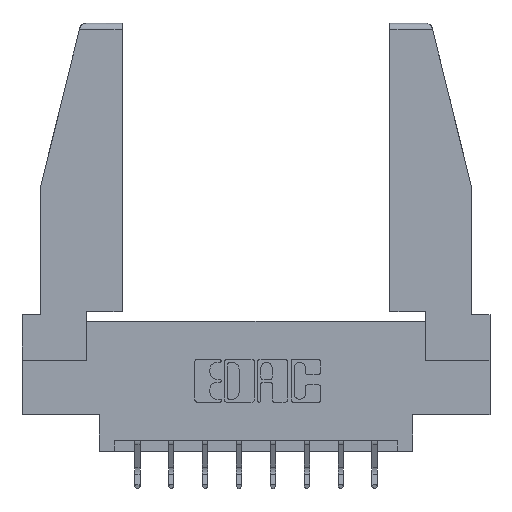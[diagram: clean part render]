
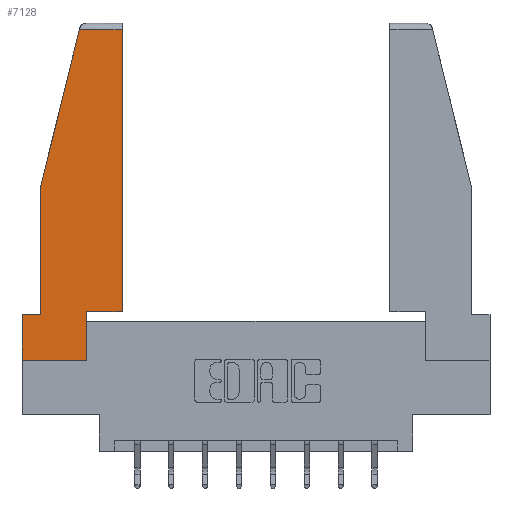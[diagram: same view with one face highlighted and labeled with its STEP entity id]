
A CAD part, top view. The second image highlights one B-rep face of the part: STEP entity #7128.
In plain terms, the highlighted planar face has unit normal (0, 0, 1).
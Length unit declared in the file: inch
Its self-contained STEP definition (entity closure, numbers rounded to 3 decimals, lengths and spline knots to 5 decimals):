
#110 = CARTESIAN_POINT ( 'NONE',  ( 0., 0.21, 0. ) ) ;
#155 = DIRECTION ( 'NONE',  ( 0., 0., 1. ) ) ;
#453 = DIRECTION ( 'NONE',  ( -1., 0., 0. ) ) ;
#784 = LINE ( 'NONE', #9707, #3025 ) ;
#1427 = VECTOR ( 'NONE', #5321, 39.37008 ) ;
#1780 = ORIENTED_EDGE ( 'NONE', *, *, #3735, .T. ) ;
#1814 = CARTESIAN_POINT ( 'NONE',  ( 0.086, 0.8, 0. ) ) ;
#1915 = ORIENTED_EDGE ( 'NONE', *, *, #5568, .T. ) ;
#1966 = CARTESIAN_POINT ( 'NONE',  ( 0.297, 0., 0. ) ) ;
#2128 = CARTESIAN_POINT ( 'NONE',  ( 0., 0., 0. ) ) ;
#2134 = VECTOR ( 'NONE', #453, 39.37008 ) ;
#2624 = CARTESIAN_POINT ( 'NONE',  ( 0.297, 0.223, 0. ) ) ;
#2722 = ORIENTED_EDGE ( 'NONE', *, *, #8441, .T. ) ;
#2969 = DIRECTION ( 'NONE',  ( -0.239, -0.971, 0. ) ) ;
#3025 = VECTOR ( 'NONE', #11882, 39.37008 ) ;
#3136 = ORIENTED_EDGE ( 'NONE', *, *, #3678, .T. ) ;
#3155 = CARTESIAN_POINT ( 'NONE',  ( 0.461, 1.52, 0. ) ) ;
#3429 = VECTOR ( 'NONE', #5223, 39.37008 ) ;
#3678 = EDGE_CURVE ( 'NONE', #12429, #12611, #9655, .T. ) ;
#3735 = EDGE_CURVE ( 'NONE', #11083, #5837, #4334, .T. ) ;
#3738 = EDGE_CURVE ( 'NONE', #8037, #12537, #784, .T. ) ;
#3771 = LINE ( 'NONE', #5772, #4568 ) ;
#3774 = VERTEX_POINT ( 'NONE', #2624 ) ;
#4039 = CARTESIAN_POINT ( 'NONE',  ( 0.086, 0.21, 0. ) ) ;
#4272 = ORIENTED_EDGE ( 'NONE', *, *, #3738, .T. ) ;
#4292 = CARTESIAN_POINT ( 'NONE',  ( 0., 0., 0. ) ) ;
#4334 = LINE ( 'NONE', #5725, #8720 ) ;
#4431 = ORIENTED_EDGE ( 'NONE', *, *, #6091, .T. ) ;
#4568 = VECTOR ( 'NONE', #6870, 39.37008 ) ;
#4651 = DIRECTION ( 'NONE',  ( 0., 1., 0. ) ) ;
#4884 = LINE ( 'NONE', #110, #2134 ) ;
#5059 = CARTESIAN_POINT ( 'NONE',  ( 0.271, 1.55, 0. ) ) ;
#5223 = DIRECTION ( 'NONE',  ( -1., 0., 0. ) ) ;
#5295 = DIRECTION ( 'NONE',  ( 0., -1., 0. ) ) ;
#5321 = DIRECTION ( 'NONE',  ( 1., 0., 0. ) ) ;
#5568 = EDGE_CURVE ( 'NONE', #12611, #3774, #3771, .T. ) ;
#5725 = CARTESIAN_POINT ( 'NONE',  ( 0.461, 0.223, 0. ) ) ;
#5772 = CARTESIAN_POINT ( 'NONE',  ( 0.297, 0., 0. ) ) ;
#5837 = VERTEX_POINT ( 'NONE', #3155 ) ;
#5842 = EDGE_CURVE ( 'NONE', #12537, #5887, #4884, .T. ) ;
#5887 = VERTEX_POINT ( 'NONE', #6706 ) ;
#6091 = EDGE_CURVE ( 'NONE', #5837, #6776, #6156, .T. ) ;
#6156 = LINE ( 'NONE', #7225, #3429 ) ;
#6706 = CARTESIAN_POINT ( 'NONE',  ( 0., 0.21, 0. ) ) ;
#6776 = VERTEX_POINT ( 'NONE', #9005 ) ;
#6785 = CARTESIAN_POINT ( 'NONE',  ( 0.461, 0.223, 0. ) ) ;
#6870 = DIRECTION ( 'NONE',  ( 0., 1., 0. ) ) ;
#6953 = VECTOR ( 'NONE', #5295, 39.37008 ) ;
#7059 = EDGE_CURVE ( 'NONE', #6776, #8037, #7287, .T. ) ;
#7128 = ADVANCED_FACE ( 'NONE', ( #7623 ), #7373, .T. ) ;
#7225 = CARTESIAN_POINT ( 'NONE',  ( 0., 1.52, 0. ) ) ;
#7287 = LINE ( 'NONE', #5059, #10402 ) ;
#7373 = PLANE ( 'NONE',  #10203 ) ;
#7623 = FACE_OUTER_BOUND ( 'NONE', #12329, .T. ) ;
#8037 = VERTEX_POINT ( 'NONE', #1814 ) ;
#8441 = EDGE_CURVE ( 'NONE', #5887, #12429, #10217, .T. ) ;
#8720 = VECTOR ( 'NONE', #4651, 39.37008 ) ;
#9005 = CARTESIAN_POINT ( 'NONE',  ( 0.2636, 1.52, 0. ) ) ;
#9465 = EDGE_CURVE ( 'NONE', #3774, #11083, #10187, .T. ) ;
#9519 = ORIENTED_EDGE ( 'NONE', *, *, #5842, .T. ) ;
#9655 = LINE ( 'NONE', #4292, #1427 ) ;
#9675 = CARTESIAN_POINT ( 'NONE',  ( 0.297, 0.223, 0. ) ) ;
#9707 = CARTESIAN_POINT ( 'NONE',  ( 0.086, 0.8, 0. ) ) ;
#9990 = ORIENTED_EDGE ( 'NONE', *, *, #9465, .T. ) ;
#10187 = LINE ( 'NONE', #9675, #11639 ) ;
#10203 = AXIS2_PLACEMENT_3D ( 'NONE', #2128, #155, #12603 ) ;
#10217 = LINE ( 'NONE', #10647, #6953 ) ;
#10402 = VECTOR ( 'NONE', #2969, 39.37008 ) ;
#10647 = CARTESIAN_POINT ( 'NONE',  ( 0., 0.21, 0. ) ) ;
#10849 = ORIENTED_EDGE ( 'NONE', *, *, #7059, .T. ) ;
#11083 = VERTEX_POINT ( 'NONE', #6785 ) ;
#11639 = VECTOR ( 'NONE', #12798, 39.37008 ) ;
#11882 = DIRECTION ( 'NONE',  ( 0., -1., 0. ) ) ;
#12329 = EDGE_LOOP ( 'NONE', ( #1780, #4431, #10849, #4272, #9519, #2722, #3136, #1915, #9990 ) ) ;
#12429 = VERTEX_POINT ( 'NONE', #12562 ) ;
#12537 = VERTEX_POINT ( 'NONE', #4039 ) ;
#12562 = CARTESIAN_POINT ( 'NONE',  ( 0., 0., 0. ) ) ;
#12603 = DIRECTION ( 'NONE',  ( 1., 0., 0. ) ) ;
#12611 = VERTEX_POINT ( 'NONE', #1966 ) ;
#12798 = DIRECTION ( 'NONE',  ( 1., 0., 0. ) ) ;
